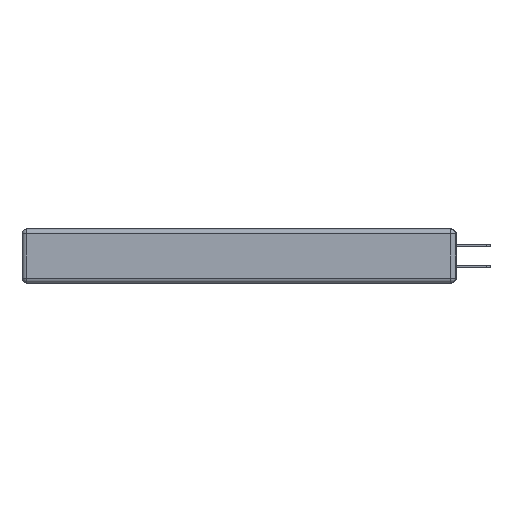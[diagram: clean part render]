
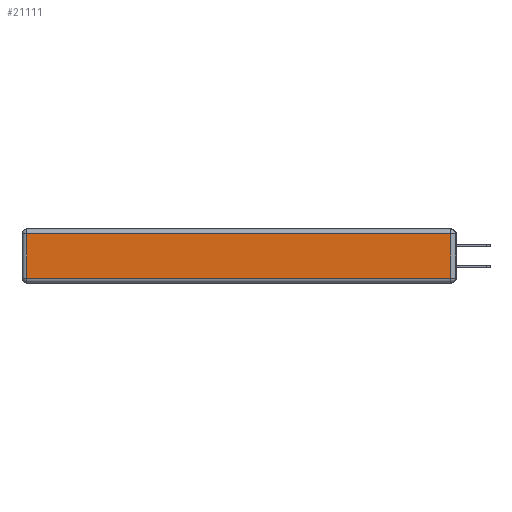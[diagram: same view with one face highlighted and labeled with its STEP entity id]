
A CAD part, left-side view. The second image highlights one B-rep face of the part: STEP entity #21111.
In plain terms, the highlighted planar face has unit normal (-1, 0, 0).
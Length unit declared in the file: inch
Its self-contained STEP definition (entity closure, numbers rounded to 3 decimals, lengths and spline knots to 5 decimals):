
#497 = LINE ( 'NONE', #20687, #11710 ) ;
#566 = DIRECTION ( 'NONE',  ( 0., -1., 0. ) ) ;
#1282 = ORIENTED_EDGE ( 'NONE', *, *, #26917, .T. ) ;
#2839 = VERTEX_POINT ( 'NONE', #12234 ) ;
#3024 = EDGE_LOOP ( 'NONE', ( #22926, #1282, #26949, #23823 ) ) ;
#3826 = DIRECTION ( 'NONE',  ( 0., 0., 1. ) ) ;
#4442 = VECTOR ( 'NONE', #566, 39.37008 ) ;
#4786 = FACE_OUTER_BOUND ( 'NONE', #3024, .T. ) ;
#6590 = VERTEX_POINT ( 'NONE', #6646 ) ;
#6646 = CARTESIAN_POINT ( 'NONE',  ( 0., 2.72, -0.313 ) ) ;
#8050 = VECTOR ( 'NONE', #3826, 39.37008 ) ;
#9127 = VERTEX_POINT ( 'NONE', #14072 ) ;
#9306 = VECTOR ( 'NONE', #10321, 39.37008 ) ;
#10214 = CARTESIAN_POINT ( 'NONE',  ( 0., 2.75, -0.03 ) ) ;
#10321 = DIRECTION ( 'NONE',  ( 0., 1., 0. ) ) ;
#11710 = VECTOR ( 'NONE', #22970, 39.37008 ) ;
#11742 = CARTESIAN_POINT ( 'NONE',  ( 0., 0., -0.343 ) ) ;
#12234 = CARTESIAN_POINT ( 'NONE',  ( 0., 0.03, -0.03 ) ) ;
#12793 = EDGE_CURVE ( 'NONE', #6590, #9127, #22617, .T. ) ;
#13066 = EDGE_CURVE ( 'NONE', #2839, #17999, #14543, .T. ) ;
#13868 = CARTESIAN_POINT ( 'NONE',  ( 0., 0., -0.313 ) ) ;
#13874 = DIRECTION ( 'NONE',  ( 0., 0., 1. ) ) ;
#14072 = CARTESIAN_POINT ( 'NONE',  ( 0., 0.03, -0.313 ) ) ;
#14543 = LINE ( 'NONE', #10214, #9306 ) ;
#15456 = EDGE_CURVE ( 'NONE', #17999, #6590, #497, .T. ) ;
#16033 = PLANE ( 'NONE',  #23058 ) ;
#16410 = DIRECTION ( 'NONE',  ( -1., 0., 0. ) ) ;
#17078 = CARTESIAN_POINT ( 'NONE',  ( 0., 2.72, -0.03 ) ) ;
#17185 = CARTESIAN_POINT ( 'NONE',  ( 0., 0.03, -0.343 ) ) ;
#17999 = VERTEX_POINT ( 'NONE', #17078 ) ;
#20687 = CARTESIAN_POINT ( 'NONE',  ( 0., 2.72, -0.343 ) ) ;
#21111 = ADVANCED_FACE ( 'NONE', ( #4786 ), #16033, .T. ) ;
#22617 = LINE ( 'NONE', #13868, #4442 ) ;
#22926 = ORIENTED_EDGE ( 'NONE', *, *, #12793, .T. ) ;
#22970 = DIRECTION ( 'NONE',  ( 0., 0., -1. ) ) ;
#23058 = AXIS2_PLACEMENT_3D ( 'NONE', #11742, #16410, #13874 ) ;
#23823 = ORIENTED_EDGE ( 'NONE', *, *, #15456, .T. ) ;
#25183 = LINE ( 'NONE', #17185, #8050 ) ;
#26917 = EDGE_CURVE ( 'NONE', #9127, #2839, #25183, .T. ) ;
#26949 = ORIENTED_EDGE ( 'NONE', *, *, #13066, .T. ) ;
